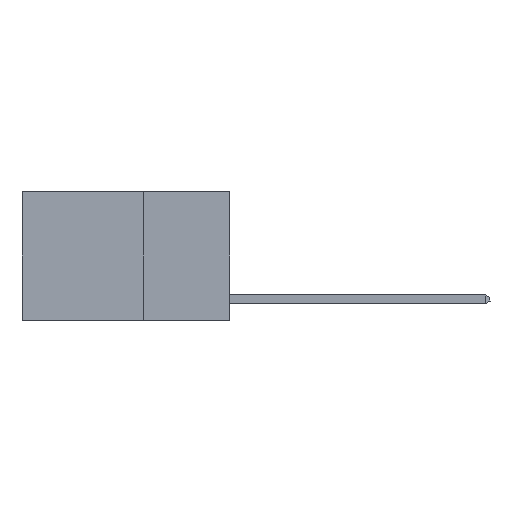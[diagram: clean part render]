
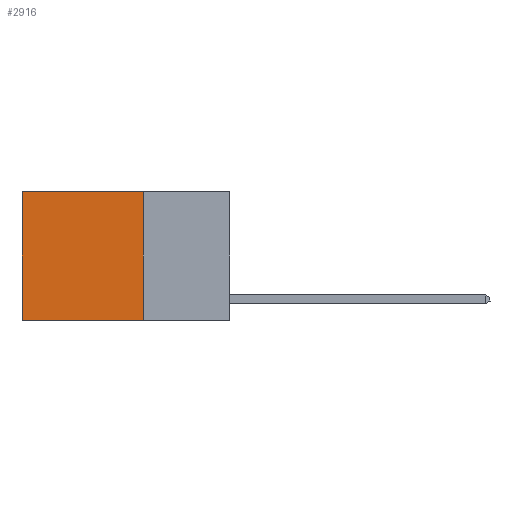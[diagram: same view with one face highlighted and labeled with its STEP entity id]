
A CAD part, left-side view. The second image highlights one B-rep face of the part: STEP entity #2916.
In plain terms, the highlighted planar face has unit normal (-1, 0, 0).
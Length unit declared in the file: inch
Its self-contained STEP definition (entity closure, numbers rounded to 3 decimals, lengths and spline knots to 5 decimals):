
#543 = AXIS2_PLACEMENT_3D ( 'NONE', #16614, #14589, #16927 ) ;
#683 = EDGE_LOOP ( 'NONE', ( #22359, #8899, #9014, #19983 ) ) ;
#2620 = CARTESIAN_POINT ( 'NONE',  ( 0.2625, 0.25, 0. ) ) ;
#2632 = LINE ( 'NONE', #18559, #16587 ) ;
#2916 = ADVANCED_FACE ( 'NONE', ( #7226 ), #4119, .F. ) ;
#3805 = VECTOR ( 'NONE', #7426, 39.37008 ) ;
#4119 = PLANE ( 'NONE',  #543 ) ;
#5461 = VERTEX_POINT ( 'NONE', #12621 ) ;
#6262 = EDGE_CURVE ( 'NONE', #5461, #8073, #2632, .T. ) ;
#6491 = VECTOR ( 'NONE', #7673, 39.37008 ) ;
#7226 = FACE_OUTER_BOUND ( 'NONE', #683, .T. ) ;
#7426 = DIRECTION ( 'NONE',  ( 0., 0., -1. ) ) ;
#7673 = DIRECTION ( 'NONE',  ( 0., 0., -1. ) ) ;
#7874 = LINE ( 'NONE', #13089, #6491 ) ;
#8073 = VERTEX_POINT ( 'NONE', #11448 ) ;
#8899 = ORIENTED_EDGE ( 'NONE', *, *, #6262, .F. ) ;
#9014 = ORIENTED_EDGE ( 'NONE', *, *, #16836, .F. ) ;
#9414 = VERTEX_POINT ( 'NONE', #19688 ) ;
#9625 = DIRECTION ( 'NONE',  ( 0., 1., 0. ) ) ;
#10924 = CARTESIAN_POINT ( 'NONE',  ( 0.2625, 0.6, 0. ) ) ;
#11342 = VECTOR ( 'NONE', #22167, 39.37008 ) ;
#11448 = CARTESIAN_POINT ( 'NONE',  ( 0.2625, 0.6, -0.37 ) ) ;
#11920 = LINE ( 'NONE', #2620, #11342 ) ;
#12612 = VERTEX_POINT ( 'NONE', #10924 ) ;
#12621 = CARTESIAN_POINT ( 'NONE',  ( 0.2625, 0.25, -0.37 ) ) ;
#13089 = CARTESIAN_POINT ( 'NONE',  ( 0.2625, 0.25, 0. ) ) ;
#14589 = DIRECTION ( 'NONE',  ( 1., 0., 0. ) ) ;
#16587 = VECTOR ( 'NONE', #9625, 39.37008 ) ;
#16614 = CARTESIAN_POINT ( 'NONE',  ( 0.2625, 0.25, 0. ) ) ;
#16836 = EDGE_CURVE ( 'NONE', #9414, #5461, #7874, .T. ) ;
#16927 = DIRECTION ( 'NONE',  ( 0., 0., -1. ) ) ;
#18095 = CARTESIAN_POINT ( 'NONE',  ( 0.2625, 0.6, 0. ) ) ;
#18559 = CARTESIAN_POINT ( 'NONE',  ( 0.2625, 0.25, -0.37 ) ) ;
#19451 = LINE ( 'NONE', #18095, #3805 ) ;
#19464 = EDGE_CURVE ( 'NONE', #12612, #8073, #19451, .T. ) ;
#19607 = EDGE_CURVE ( 'NONE', #9414, #12612, #11920, .T. ) ;
#19688 = CARTESIAN_POINT ( 'NONE',  ( 0.2625, 0.25, 0. ) ) ;
#19983 = ORIENTED_EDGE ( 'NONE', *, *, #19607, .T. ) ;
#22167 = DIRECTION ( 'NONE',  ( 0., 1., 0. ) ) ;
#22359 = ORIENTED_EDGE ( 'NONE', *, *, #19464, .T. ) ;
